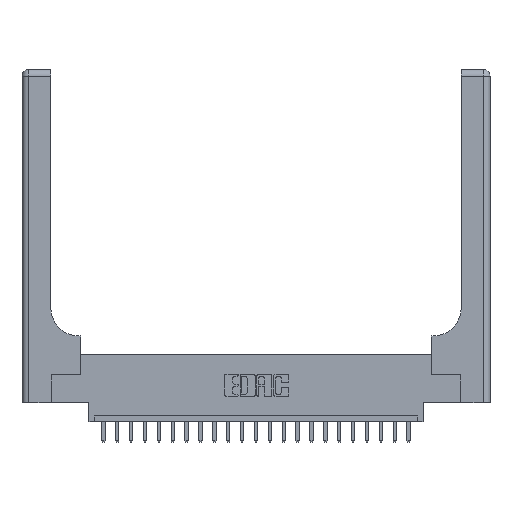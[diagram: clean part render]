
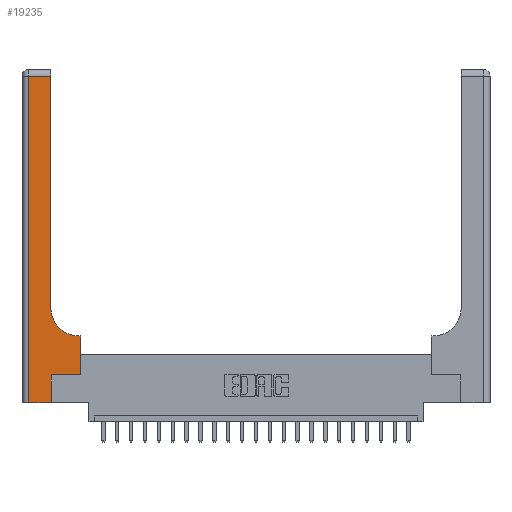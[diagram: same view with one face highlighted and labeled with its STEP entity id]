
A CAD part, top view. The second image highlights one B-rep face of the part: STEP entity #19235.
In plain terms, the highlighted planar face has unit normal (0, 0, 1).
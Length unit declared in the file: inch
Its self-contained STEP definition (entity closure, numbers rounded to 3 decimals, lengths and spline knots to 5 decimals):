
#1128 = CIRCLE ( 'NONE', #6997, 0.25 ) ;
#1400 = ORIENTED_EDGE ( 'NONE', *, *, #15508, .T. ) ;
#1519 = ORIENTED_EDGE ( 'NONE', *, *, #14709, .T. ) ;
#1848 = EDGE_CURVE ( 'NONE', #21945, #12305, #9779, .T. ) ;
#2283 = CARTESIAN_POINT ( 'NONE',  ( 0.265, 0.25, 0.37 ) ) ;
#2691 = ORIENTED_EDGE ( 'NONE', *, *, #1848, .T. ) ;
#3146 = VECTOR ( 'NONE', #8340, 39.37008 ) ;
#3552 = DIRECTION ( 'NONE',  ( -1., 0., 0. ) ) ;
#3611 = VERTEX_POINT ( 'NONE', #12980 ) ;
#3778 = DIRECTION ( 'NONE',  ( -1., 0., 0. ) ) ;
#4037 = CARTESIAN_POINT ( 'NONE',  ( 0.06, 0., 0.37 ) ) ;
#4134 = EDGE_CURVE ( 'NONE', #15970, #17026, #18351, .T. ) ;
#4257 = LINE ( 'NONE', #13402, #17480 ) ;
#4282 = DIRECTION ( 'NONE',  ( -1., 0., 0. ) ) ;
#4949 = DIRECTION ( 'NONE',  ( 0., 0., -1. ) ) ;
#5019 = VECTOR ( 'NONE', #17742, 39.37008 ) ;
#5176 = EDGE_LOOP ( 'NONE', ( #1400, #2691, #19186, #8277, #14586, #14142, #1519, #10738, #10152 ) ) ;
#5434 = LINE ( 'NONE', #12422, #16749 ) ;
#5820 = LINE ( 'NONE', #9488, #5019 ) ;
#6324 = DIRECTION ( 'NONE',  ( 0., 1., 0. ) ) ;
#6348 = CARTESIAN_POINT ( 'NONE',  ( 0.528, 0.25, 0.37 ) ) ;
#6997 = AXIS2_PLACEMENT_3D ( 'NONE', #17611, #9242, #12897 ) ;
#7068 = LINE ( 'NONE', #18991, #3146 ) ;
#7091 = CARTESIAN_POINT ( 'NONE',  ( 0., 0., 0.37 ) ) ;
#7227 = CARTESIAN_POINT ( 'NONE',  ( 0., 3., 0.37 ) ) ;
#7767 = CARTESIAN_POINT ( 'NONE',  ( 0.51, 0.6, 0.37 ) ) ;
#7854 = EDGE_CURVE ( 'NONE', #10171, #14765, #1128, .T. ) ;
#8277 = ORIENTED_EDGE ( 'NONE', *, *, #11836, .T. ) ;
#8340 = DIRECTION ( 'NONE',  ( 0., -1., 0. ) ) ;
#8508 = PLANE ( 'NONE',  #18643 ) ;
#9242 = DIRECTION ( 'NONE',  ( 0., 0., -1. ) ) ;
#9488 = CARTESIAN_POINT ( 'NONE',  ( 0.528, 0.25, 0.37 ) ) ;
#9773 = CARTESIAN_POINT ( 'NONE',  ( 0.06, 2.94, 0.37 ) ) ;
#9779 = LINE ( 'NONE', #15032, #16907 ) ;
#10152 = ORIENTED_EDGE ( 'NONE', *, *, #7854, .T. ) ;
#10171 = VERTEX_POINT ( 'NONE', #7767 ) ;
#10528 = LINE ( 'NONE', #7091, #12248 ) ;
#10738 = ORIENTED_EDGE ( 'NONE', *, *, #18305, .T. ) ;
#10883 = LINE ( 'NONE', #17991, #17863 ) ;
#10955 = VERTEX_POINT ( 'NONE', #4037 ) ;
#10975 = CARTESIAN_POINT ( 'NONE',  ( 0.26, 0.85, 0.37 ) ) ;
#11836 = EDGE_CURVE ( 'NONE', #10955, #3611, #10528, .T. ) ;
#12177 = FACE_OUTER_BOUND ( 'NONE', #5176, .T. ) ;
#12248 = VECTOR ( 'NONE', #17735, 39.37008 ) ;
#12305 = VERTEX_POINT ( 'NONE', #9773 ) ;
#12422 = CARTESIAN_POINT ( 'NONE',  ( 0.26, 3., 0.37 ) ) ;
#12897 = DIRECTION ( 'NONE',  ( 1., 0., 0. ) ) ;
#12980 = CARTESIAN_POINT ( 'NONE',  ( 0.265, 0., 0.37 ) ) ;
#13400 = CARTESIAN_POINT ( 'NONE',  ( 0.265, 0.25, 0.37 ) ) ;
#13402 = CARTESIAN_POINT ( 'NONE',  ( 0.265, 0., 0.37 ) ) ;
#13772 = CARTESIAN_POINT ( 'NONE',  ( 0.528, 0.6, 0.37 ) ) ;
#13810 = EDGE_CURVE ( 'NONE', #12305, #10955, #7068, .T. ) ;
#14142 = ORIENTED_EDGE ( 'NONE', *, *, #4134, .T. ) ;
#14586 = ORIENTED_EDGE ( 'NONE', *, *, #17446, .T. ) ;
#14709 = EDGE_CURVE ( 'NONE', #17026, #17217, #5820, .T. ) ;
#14765 = VERTEX_POINT ( 'NONE', #10975 ) ;
#15032 = CARTESIAN_POINT ( 'NONE',  ( 0., 2.94, 0.37 ) ) ;
#15508 = EDGE_CURVE ( 'NONE', #14765, #21945, #5434, .T. ) ;
#15970 = VERTEX_POINT ( 'NONE', #2283 ) ;
#16629 = DIRECTION ( 'NONE',  ( 1., 0., 0. ) ) ;
#16749 = VECTOR ( 'NONE', #19765, 39.37008 ) ;
#16907 = VECTOR ( 'NONE', #4282, 39.37008 ) ;
#17026 = VERTEX_POINT ( 'NONE', #6348 ) ;
#17217 = VERTEX_POINT ( 'NONE', #13772 ) ;
#17446 = EDGE_CURVE ( 'NONE', #3611, #15970, #4257, .T. ) ;
#17480 = VECTOR ( 'NONE', #6324, 39.37008 ) ;
#17611 = CARTESIAN_POINT ( 'NONE',  ( 0.51, 0.85, 0.37 ) ) ;
#17735 = DIRECTION ( 'NONE',  ( 1., 0., 0. ) ) ;
#17742 = DIRECTION ( 'NONE',  ( 0., 1., 0. ) ) ;
#17863 = VECTOR ( 'NONE', #3778, 39.37008 ) ;
#17991 = CARTESIAN_POINT ( 'NONE',  ( 0.26, 0.6, 0.37 ) ) ;
#18305 = EDGE_CURVE ( 'NONE', #17217, #10171, #10883, .T. ) ;
#18351 = LINE ( 'NONE', #13400, #19969 ) ;
#18643 = AXIS2_PLACEMENT_3D ( 'NONE', #7227, #4949, #3552 ) ;
#18991 = CARTESIAN_POINT ( 'NONE',  ( 0.06, 3., 0.37 ) ) ;
#19070 = CARTESIAN_POINT ( 'NONE',  ( 0.26, 2.94, 0.37 ) ) ;
#19186 = ORIENTED_EDGE ( 'NONE', *, *, #13810, .T. ) ;
#19235 = ADVANCED_FACE ( 'NONE', ( #12177 ), #8508, .F. ) ;
#19765 = DIRECTION ( 'NONE',  ( 0., 1., 0. ) ) ;
#19969 = VECTOR ( 'NONE', #16629, 39.37008 ) ;
#21945 = VERTEX_POINT ( 'NONE', #19070 ) ;
